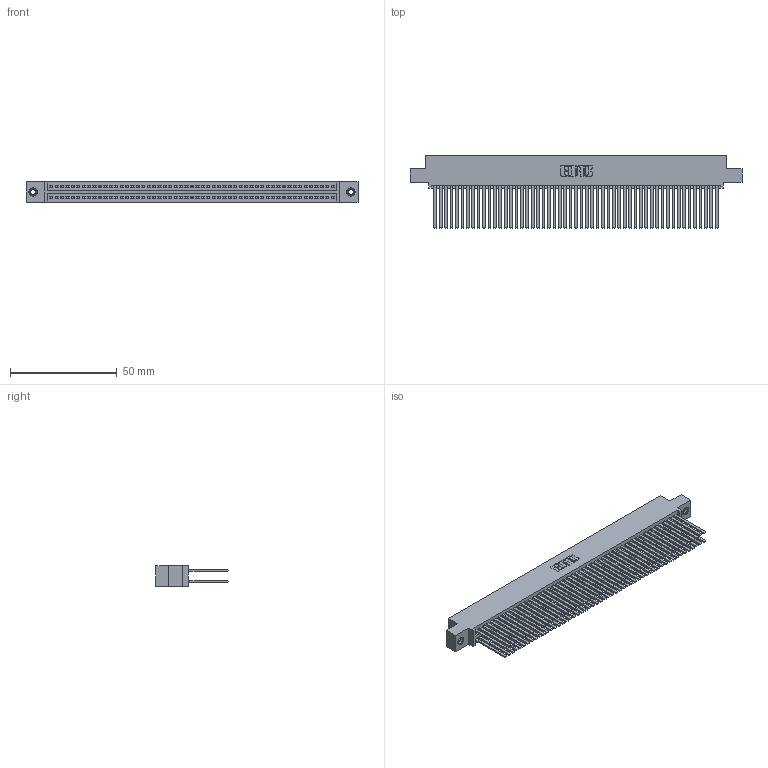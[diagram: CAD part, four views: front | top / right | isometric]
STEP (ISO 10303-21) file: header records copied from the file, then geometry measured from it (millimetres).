
FILE_DESCRIPTION (( 'STEP AP203' ), '1' );
FILE_NAME ('345-106-544-508.STEP', '2019-11-03T16:44:13', ( '' ), ( '' ), 'SwSTEP 2.0', 'SolidWorks 2016', '' );
FILE_SCHEMA (( 'CONFIG_CONTROL_DESIGN' ));
Length unit declared in the file: inch
Products named in the file (4): 345-250-001_345-250-003-102; 345-292-001_345-293-144; 345-106-544-508; 345 Part_0.110 Offset - 0.156 Dia-TI
Assembly tree (109 placements, depth 2):
  345-106-544-508
    345 Part_0.110 Offset - 0.156 Dia-TI
    345-292-001_345-293-144  x106
    345-250-001_345-250-003-102  x2
Bounding box: 155.83 x 33.96 x 9.4 mm (x, y, z)
Volume: 16645.5 mm3; surface area: 29279.3 mm2
Topology: 109 solids, 109 shells, 4854 faces, 14375 edges, 9434 vertices
Faces by surface type: plane 3190, cylinder 1648, cone 12, torus 4
Entity records: 41238 total; most frequent: CARTESIAN_POINT 6883, ORIENTED_EDGE 6810, DIRECTION 6079, EDGE_CURVE 3405, VECTOR 3045, LINE 3045, VERTEX_POINT 2264, AXIS2_PLACEMENT_3D 1517
